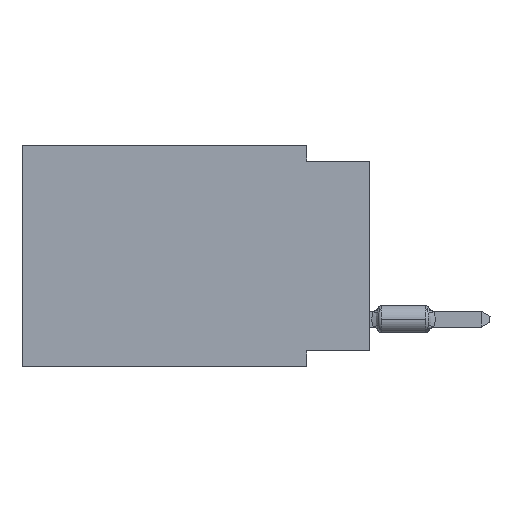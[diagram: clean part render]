
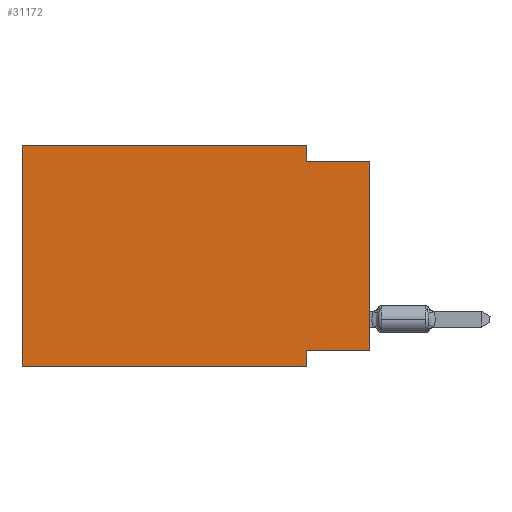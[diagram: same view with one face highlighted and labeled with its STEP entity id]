
A CAD part, left-side view. The second image highlights one B-rep face of the part: STEP entity #31172.
In plain terms, the highlighted planar face has unit normal (-1, 0, 0).
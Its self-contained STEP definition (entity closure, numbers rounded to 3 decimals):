
#796 = EDGE_CURVE ( 'NONE', #35032, #36077, #849, .T. ) ;
#849 = LINE ( 'NONE', #15446, #32319 ) ;
#946 = CARTESIAN_POINT ( 'NONE',  ( 0., 0., -0.635 ) ) ;
#1129 = LINE ( 'NONE', #946, #38601 ) ;
#1710 = LINE ( 'NONE', #16738, #17826 ) ;
#2125 = CARTESIAN_POINT ( 'NONE',  ( 0., 2.54, -0.635 ) ) ;
#2866 = VERTEX_POINT ( 'NONE', #14903 ) ;
#3121 = ORIENTED_EDGE ( 'NONE', *, *, #15091, .F. ) ;
#3210 = CARTESIAN_POINT ( 'NONE',  ( 0., 13.97, 0. ) ) ;
#3406 = DIRECTION ( 'NONE',  ( 0., -1., 0. ) ) ;
#4182 = EDGE_CURVE ( 'NONE', #25395, #23965, #36081, .T. ) ;
#4369 = CARTESIAN_POINT ( 'NONE',  ( 0., 13.97, 0. ) ) ;
#5792 = LINE ( 'NONE', #3210, #25760 ) ;
#6133 = LINE ( 'NONE', #18177, #14595 ) ;
#6637 = EDGE_CURVE ( 'NONE', #20202, #36077, #7542, .T. ) ;
#7152 = DIRECTION ( 'NONE',  ( 1., 0., 0. ) ) ;
#7542 = LINE ( 'NONE', #29052, #38411 ) ;
#7562 = VECTOR ( 'NONE', #38471, 1000. ) ;
#9164 = EDGE_CURVE ( 'NONE', #2866, #20202, #6133, .T. ) ;
#9816 = DIRECTION ( 'NONE',  ( 0., -1., 0. ) ) ;
#12412 = CARTESIAN_POINT ( 'NONE',  ( 0., 2.54, -8.255 ) ) ;
#13256 = DIRECTION ( 'NONE',  ( 0., 0., -1. ) ) ;
#14595 = VECTOR ( 'NONE', #32584, 1000. ) ;
#14903 = CARTESIAN_POINT ( 'NONE',  ( 0., 0., -8.255 ) ) ;
#15091 = EDGE_CURVE ( 'NONE', #23965, #38822, #1129, .T. ) ;
#15446 = CARTESIAN_POINT ( 'NONE',  ( 0., 13.97, -8.89 ) ) ;
#15787 = EDGE_CURVE ( 'NONE', #37163, #25395, #5792, .T. ) ;
#16626 = ORIENTED_EDGE ( 'NONE', *, *, #9164, .F. ) ;
#16738 = CARTESIAN_POINT ( 'NONE',  ( 0., 0., 0. ) ) ;
#16907 = VECTOR ( 'NONE', #35417, 1000. ) ;
#17640 = CARTESIAN_POINT ( 'NONE',  ( 0., 13.97, 0. ) ) ;
#17826 = VECTOR ( 'NONE', #32105, 1000. ) ;
#18177 = CARTESIAN_POINT ( 'NONE',  ( 0., 0., -8.255 ) ) ;
#19589 = DIRECTION ( 'NONE',  ( 0., 0., -1. ) ) ;
#20015 = CARTESIAN_POINT ( 'NONE',  ( 0., 2.54, 0. ) ) ;
#20202 = VERTEX_POINT ( 'NONE', #12412 ) ;
#20427 = LINE ( 'NONE', #17640, #16907 ) ;
#20606 = CARTESIAN_POINT ( 'NONE',  ( 0., 13.97, -8.89 ) ) ;
#20868 = AXIS2_PLACEMENT_3D ( 'NONE', #4369, #7152, #13256 ) ;
#20890 = CARTESIAN_POINT ( 'NONE',  ( 0., 2.54, 0. ) ) ;
#21181 = ORIENTED_EDGE ( 'NONE', *, *, #6637, .F. ) ;
#22607 = EDGE_CURVE ( 'NONE', #2866, #38822, #1710, .T. ) ;
#23965 = VERTEX_POINT ( 'NONE', #2125 ) ;
#24169 = CARTESIAN_POINT ( 'NONE',  ( 0., 0., -0.635 ) ) ;
#24873 = ORIENTED_EDGE ( 'NONE', *, *, #26510, .F. ) ;
#25309 = FACE_OUTER_BOUND ( 'NONE', #37957, .T. ) ;
#25395 = VERTEX_POINT ( 'NONE', #20015 ) ;
#25760 = VECTOR ( 'NONE', #32618, 1000. ) ;
#26124 = ORIENTED_EDGE ( 'NONE', *, *, #4182, .F. ) ;
#26510 = EDGE_CURVE ( 'NONE', #35032, #37163, #20427, .T. ) ;
#28836 = PLANE ( 'NONE',  #20868 ) ;
#29052 = CARTESIAN_POINT ( 'NONE',  ( 0., 2.54, -8.89 ) ) ;
#29071 = ORIENTED_EDGE ( 'NONE', *, *, #796, .T. ) ;
#29133 = CARTESIAN_POINT ( 'NONE',  ( 0., 2.54, -8.89 ) ) ;
#31172 = ADVANCED_FACE ( 'NONE', ( #25309 ), #28836, .F. ) ;
#31550 = ORIENTED_EDGE ( 'NONE', *, *, #15787, .F. ) ;
#32105 = DIRECTION ( 'NONE',  ( 0., 0., 1. ) ) ;
#32319 = VECTOR ( 'NONE', #3406, 1000. ) ;
#32584 = DIRECTION ( 'NONE',  ( 0., 1., 0. ) ) ;
#32618 = DIRECTION ( 'NONE',  ( 0., -1., 0. ) ) ;
#33685 = ORIENTED_EDGE ( 'NONE', *, *, #22607, .T. ) ;
#35032 = VERTEX_POINT ( 'NONE', #20606 ) ;
#35417 = DIRECTION ( 'NONE',  ( 0., 0., 1. ) ) ;
#36077 = VERTEX_POINT ( 'NONE', #29133 ) ;
#36081 = LINE ( 'NONE', #20890, #7562 ) ;
#36644 = CARTESIAN_POINT ( 'NONE',  ( 0., 13.97, 0. ) ) ;
#37163 = VERTEX_POINT ( 'NONE', #36644 ) ;
#37957 = EDGE_LOOP ( 'NONE', ( #33685, #3121, #26124, #31550, #24873, #29071, #21181, #16626 ) ) ;
#38411 = VECTOR ( 'NONE', #19589, 1000. ) ;
#38471 = DIRECTION ( 'NONE',  ( 0., 0., -1. ) ) ;
#38601 = VECTOR ( 'NONE', #9816, 1000. ) ;
#38822 = VERTEX_POINT ( 'NONE', #24169 ) ;
